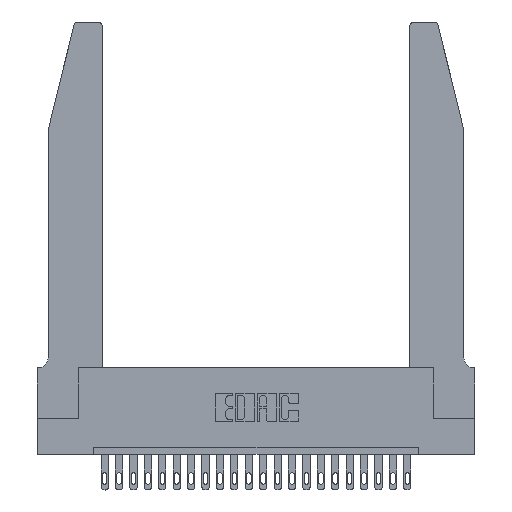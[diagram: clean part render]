
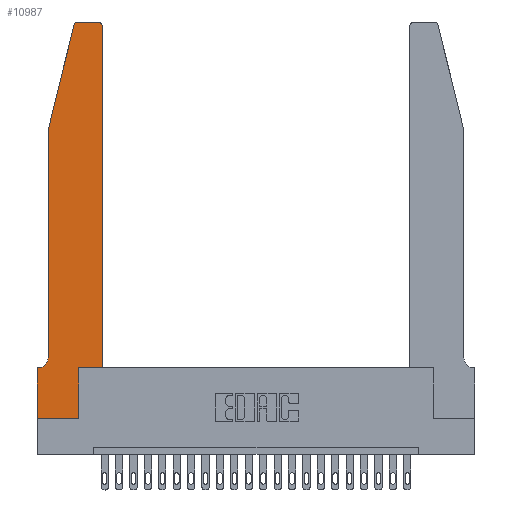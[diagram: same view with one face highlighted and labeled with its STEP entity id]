
A CAD part, top view. The second image highlights one B-rep face of the part: STEP entity #10987.
In plain terms, the highlighted planar face has unit normal (0, 0, 1).
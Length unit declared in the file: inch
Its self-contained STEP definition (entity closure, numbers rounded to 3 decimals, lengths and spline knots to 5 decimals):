
#268 = LINE ( 'NONE', #22667, #1448 ) ;
#523 = EDGE_CURVE ( 'NONE', #13821, #5047, #8827, .T. ) ;
#930 = AXIS2_PLACEMENT_3D ( 'NONE', #22127, #20221, #3747 ) ;
#1369 = FACE_OUTER_BOUND ( 'NONE', #23870, .T. ) ;
#1448 = VECTOR ( 'NONE', #22497, 39.37008 ) ;
#1505 = VERTEX_POINT ( 'NONE', #1864 ) ;
#1722 = DIRECTION ( 'NONE',  ( 0., 0., 1. ) ) ;
#1864 = CARTESIAN_POINT ( 'NONE',  ( 0., 0.35, 0.37 ) ) ;
#2313 = CARTESIAN_POINT ( 'NONE',  ( 0., 0., 0.37 ) ) ;
#2360 = LINE ( 'NONE', #3033, #9658 ) ;
#2541 = VERTEX_POINT ( 'NONE', #7726 ) ;
#2877 = DIRECTION ( 'NONE',  ( 0., 0., 1. ) ) ;
#3033 = CARTESIAN_POINT ( 'NONE',  ( 0.4505, 0.35, 0.37 ) ) ;
#3282 = CARTESIAN_POINT ( 'NONE',  ( 0.4505, 0.35, 0.37 ) ) ;
#3390 = CARTESIAN_POINT ( 'NONE',  ( 0., 0., 0.37 ) ) ;
#3447 = DIRECTION ( 'NONE',  ( 0., 0., -1. ) ) ;
#3747 = DIRECTION ( 'NONE',  ( 1., 0., 0. ) ) ;
#3903 = LINE ( 'NONE', #15388, #9162 ) ;
#4133 = VECTOR ( 'NONE', #6253, 39.37008 ) ;
#4226 = CIRCLE ( 'NONE', #12631, 0.07 ) ;
#4376 = ORIENTED_EDGE ( 'NONE', *, *, #10635, .T. ) ;
#4551 = VERTEX_POINT ( 'NONE', #4985 ) ;
#4808 = CARTESIAN_POINT ( 'NONE',  ( 0.4505, 2.72, 0.37 ) ) ;
#4903 = VECTOR ( 'NONE', #11217, 39.37008 ) ;
#4985 = CARTESIAN_POINT ( 'NONE',  ( 0.0755, 0.42, 0.37 ) ) ;
#5047 = VERTEX_POINT ( 'NONE', #14669 ) ;
#5108 = ORIENTED_EDGE ( 'NONE', *, *, #5275, .T. ) ;
#5275 = EDGE_CURVE ( 'NONE', #14495, #2541, #17572, .T. ) ;
#5343 = EDGE_CURVE ( 'NONE', #4551, #20061, #4226, .T. ) ;
#5392 = DIRECTION ( 'NONE',  ( 1., 0., 0. ) ) ;
#5879 = AXIS2_PLACEMENT_3D ( 'NONE', #10778, #1722, #5392 ) ;
#5998 = ORIENTED_EDGE ( 'NONE', *, *, #7557, .T. ) ;
#6253 = DIRECTION ( 'NONE',  ( 1., 0., 0. ) ) ;
#6496 = DIRECTION ( 'NONE',  ( -1., 0., 0. ) ) ;
#6979 = EDGE_CURVE ( 'NONE', #2541, #17531, #14072, .T. ) ;
#6989 = DIRECTION ( 'NONE',  ( 1., 0., 0. ) ) ;
#7260 = ORIENTED_EDGE ( 'NONE', *, *, #21718, .T. ) ;
#7557 = EDGE_CURVE ( 'NONE', #8209, #13755, #2360, .T. ) ;
#7726 = CARTESIAN_POINT ( 'NONE',  ( 0.25487, 2.72718, 0.37 ) ) ;
#7757 = ORIENTED_EDGE ( 'NONE', *, *, #22892, .T. ) ;
#8181 = CARTESIAN_POINT ( 'NONE',  ( 0., 0., 0.37 ) ) ;
#8209 = VERTEX_POINT ( 'NONE', #15303 ) ;
#8419 = VECTOR ( 'NONE', #22426, 39.37008 ) ;
#8499 = CARTESIAN_POINT ( 'NONE',  ( 0.0055, 0.35, 0.37 ) ) ;
#8564 = VECTOR ( 'NONE', #16324, 39.37008 ) ;
#8643 = CARTESIAN_POINT ( 'NONE',  ( 0.0755, 2., 0.37 ) ) ;
#8827 = CIRCLE ( 'NONE', #930, 0.03 ) ;
#9136 = ORIENTED_EDGE ( 'NONE', *, *, #22790, .T. ) ;
#9162 = VECTOR ( 'NONE', #21098, 39.37008 ) ;
#9622 = EDGE_CURVE ( 'NONE', #18918, #8209, #12455, .T. ) ;
#9658 = VECTOR ( 'NONE', #6989, 39.37008 ) ;
#10004 = LINE ( 'NONE', #2313, #4133 ) ;
#10351 = CARTESIAN_POINT ( 'NONE',  ( 0.0055, 0.42, 0.37 ) ) ;
#10635 = EDGE_CURVE ( 'NONE', #17531, #4551, #21393, .T. ) ;
#10778 = CARTESIAN_POINT ( 'NONE',  ( 0., 0.35, 0.37 ) ) ;
#10987 = ADVANCED_FACE ( 'NONE', ( #1369 ), #13971, .T. ) ;
#11217 = DIRECTION ( 'NONE',  ( 0., 1., 0. ) ) ;
#12104 = DIRECTION ( 'NONE',  ( -0.239, -0.971, 0. ) ) ;
#12455 = LINE ( 'NONE', #16821, #4903 ) ;
#12531 = EDGE_CURVE ( 'NONE', #5047, #14495, #14408, .T. ) ;
#12631 = AXIS2_PLACEMENT_3D ( 'NONE', #10351, #3447, #23797 ) ;
#13335 = EDGE_CURVE ( 'NONE', #20061, #1505, #268, .T. ) ;
#13755 = VERTEX_POINT ( 'NONE', #3282 ) ;
#13821 = VERTEX_POINT ( 'NONE', #4808 ) ;
#13868 = DIRECTION ( 'NONE',  ( 1., 0., 0. ) ) ;
#13877 = ORIENTED_EDGE ( 'NONE', *, *, #13335, .T. ) ;
#13893 = AXIS2_PLACEMENT_3D ( 'NONE', #14033, #2877, #13868 ) ;
#13971 = PLANE ( 'NONE',  #5879 ) ;
#14026 = CARTESIAN_POINT ( 'NONE',  ( 0.2605, 2.75, 0.37 ) ) ;
#14033 = CARTESIAN_POINT ( 'NONE',  ( 0.284, 2.72, 0.37 ) ) ;
#14072 = LINE ( 'NONE', #8643, #19536 ) ;
#14408 = LINE ( 'NONE', #14026, #17535 ) ;
#14495 = VERTEX_POINT ( 'NONE', #20499 ) ;
#14648 = LINE ( 'NONE', #3390, #8564 ) ;
#14669 = CARTESIAN_POINT ( 'NONE',  ( 0.4205, 2.75, 0.37 ) ) ;
#15303 = CARTESIAN_POINT ( 'NONE',  ( 0.2865, 0.35, 0.37 ) ) ;
#15388 = CARTESIAN_POINT ( 'NONE',  ( 0.4505, 0.35, 0.37 ) ) ;
#16324 = DIRECTION ( 'NONE',  ( 0., -1., 0. ) ) ;
#16821 = CARTESIAN_POINT ( 'NONE',  ( 0.2865, 0.35, 0.37 ) ) ;
#17531 = VERTEX_POINT ( 'NONE', #20306 ) ;
#17535 = VECTOR ( 'NONE', #6496, 39.37008 ) ;
#17557 = CARTESIAN_POINT ( 'NONE',  ( 0.2865, 0., 0.37 ) ) ;
#17572 = CIRCLE ( 'NONE', #13893, 0.03 ) ;
#18174 = ORIENTED_EDGE ( 'NONE', *, *, #9622, .T. ) ;
#18918 = VERTEX_POINT ( 'NONE', #17557 ) ;
#19536 = VECTOR ( 'NONE', #12104, 39.37008 ) ;
#20061 = VERTEX_POINT ( 'NONE', #8499 ) ;
#20221 = DIRECTION ( 'NONE',  ( 0., 0., 1. ) ) ;
#20306 = CARTESIAN_POINT ( 'NONE',  ( 0.0755, 2., 0.37 ) ) ;
#20317 = ORIENTED_EDGE ( 'NONE', *, *, #5343, .T. ) ;
#20499 = CARTESIAN_POINT ( 'NONE',  ( 0.284, 2.75, 0.37 ) ) ;
#21098 = DIRECTION ( 'NONE',  ( 0., 1., 0. ) ) ;
#21393 = LINE ( 'NONE', #22599, #8419 ) ;
#21718 = EDGE_CURVE ( 'NONE', #13755, #13821, #3903, .T. ) ;
#21869 = VERTEX_POINT ( 'NONE', #8181 ) ;
#22127 = CARTESIAN_POINT ( 'NONE',  ( 0.4205, 2.72, 0.37 ) ) ;
#22364 = ORIENTED_EDGE ( 'NONE', *, *, #6979, .T. ) ;
#22426 = DIRECTION ( 'NONE',  ( 0., -1., 0. ) ) ;
#22497 = DIRECTION ( 'NONE',  ( -1., 0., 0. ) ) ;
#22599 = CARTESIAN_POINT ( 'NONE',  ( 0.0755, 2., 0.37 ) ) ;
#22667 = CARTESIAN_POINT ( 'NONE',  ( 0.0755, 0.35, 0.37 ) ) ;
#22790 = EDGE_CURVE ( 'NONE', #1505, #21869, #14648, .T. ) ;
#22892 = EDGE_CURVE ( 'NONE', #21869, #18918, #10004, .T. ) ;
#23343 = ORIENTED_EDGE ( 'NONE', *, *, #12531, .T. ) ;
#23797 = DIRECTION ( 'NONE',  ( -1., 0., 0. ) ) ;
#23870 = EDGE_LOOP ( 'NONE', ( #23343, #5108, #22364, #4376, #20317, #13877, #9136, #7757, #18174, #5998, #7260, #23922 ) ) ;
#23922 = ORIENTED_EDGE ( 'NONE', *, *, #523, .T. ) ;
